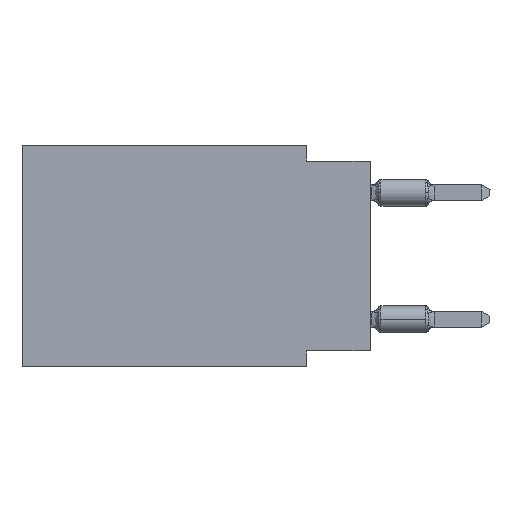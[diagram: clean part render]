
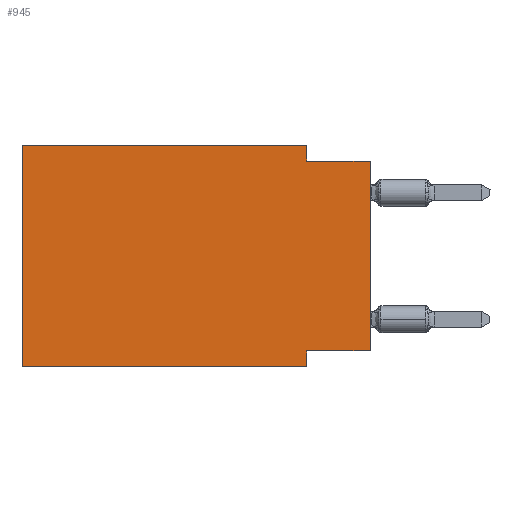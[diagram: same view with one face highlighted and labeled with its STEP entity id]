
A CAD part, left-side view. The second image highlights one B-rep face of the part: STEP entity #945.
In plain terms, the highlighted planar face has unit normal (-1, 0, 0).
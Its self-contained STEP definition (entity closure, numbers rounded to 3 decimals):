
#302 = CARTESIAN_POINT ( 'NONE',  ( 0., 13.97, 0. ) ) ;
#624 = CARTESIAN_POINT ( 'NONE',  ( 0., 0., 0. ) ) ;
#787 = VECTOR ( 'NONE', #10287, 1000. ) ;
#945 = ADVANCED_FACE ( 'NONE', ( #7167 ), #45104, .F. ) ;
#946 = ORIENTED_EDGE ( 'NONE', *, *, #25807, .F. ) ;
#1257 = CARTESIAN_POINT ( 'NONE',  ( 0., 13.97, 0. ) ) ;
#1689 = CARTESIAN_POINT ( 'NONE',  ( 0., 13.97, 0. ) ) ;
#1905 = VERTEX_POINT ( 'NONE', #18632 ) ;
#2307 = ORIENTED_EDGE ( 'NONE', *, *, #4470, .F. ) ;
#2463 = VERTEX_POINT ( 'NONE', #44255 ) ;
#2553 = CARTESIAN_POINT ( 'NONE',  ( 0., 2.54, -8.89 ) ) ;
#2844 = VERTEX_POINT ( 'NONE', #2553 ) ;
#2991 = LINE ( 'NONE', #7091, #787 ) ;
#4079 = EDGE_CURVE ( 'NONE', #14076, #1905, #31933, .T. ) ;
#4213 = ORIENTED_EDGE ( 'NONE', *, *, #28203, .F. ) ;
#4470 = EDGE_CURVE ( 'NONE', #2463, #1905, #44933, .T. ) ;
#4585 = LINE ( 'NONE', #14881, #16093 ) ;
#6773 = DIRECTION ( 'NONE',  ( 0., -1., 0. ) ) ;
#7091 = CARTESIAN_POINT ( 'NONE',  ( 0., 2.54, -8.89 ) ) ;
#7167 = FACE_OUTER_BOUND ( 'NONE', #30741, .T. ) ;
#7671 = DIRECTION ( 'NONE',  ( 0., 0., 1. ) ) ;
#9624 = VECTOR ( 'NONE', #35718, 1000. ) ;
#10287 = DIRECTION ( 'NONE',  ( 0., 0., -1. ) ) ;
#10493 = VECTOR ( 'NONE', #6773, 1000. ) ;
#10556 = VECTOR ( 'NONE', #17988, 1000. ) ;
#11600 = EDGE_CURVE ( 'NONE', #29975, #2844, #30403, .T. ) ;
#11664 = CARTESIAN_POINT ( 'NONE',  ( 0., 0., -8.255 ) ) ;
#14076 = VERTEX_POINT ( 'NONE', #11664 ) ;
#14382 = ORIENTED_EDGE ( 'NONE', *, *, #4079, .T. ) ;
#14881 = CARTESIAN_POINT ( 'NONE',  ( 0., 13.97, 0. ) ) ;
#16093 = VECTOR ( 'NONE', #35660, 1000. ) ;
#16853 = VERTEX_POINT ( 'NONE', #23059 ) ;
#17988 = DIRECTION ( 'NONE',  ( 0., 0., 1. ) ) ;
#18632 = CARTESIAN_POINT ( 'NONE',  ( 0., 0., -0.635 ) ) ;
#18939 = VERTEX_POINT ( 'NONE', #20439 ) ;
#20439 = CARTESIAN_POINT ( 'NONE',  ( 0., 2.54, 0. ) ) ;
#21323 = DIRECTION ( 'NONE',  ( 0., 0., -1. ) ) ;
#21767 = LINE ( 'NONE', #24309, #9624 ) ;
#23059 = CARTESIAN_POINT ( 'NONE',  ( 0., 2.54, -8.255 ) ) ;
#24309 = CARTESIAN_POINT ( 'NONE',  ( 0., 0., -8.255 ) ) ;
#25141 = EDGE_CURVE ( 'NONE', #29975, #31504, #32350, .T. ) ;
#25807 = EDGE_CURVE ( 'NONE', #31504, #18939, #4585, .T. ) ;
#26710 = EDGE_CURVE ( 'NONE', #18939, #2463, #34114, .T. ) ;
#27057 = ORIENTED_EDGE ( 'NONE', *, *, #11600, .T. ) ;
#27412 = CARTESIAN_POINT ( 'NONE',  ( 0., 13.97, -8.89 ) ) ;
#27734 = DIRECTION ( 'NONE',  ( 1., 0., 0. ) ) ;
#27994 = ORIENTED_EDGE ( 'NONE', *, *, #25141, .F. ) ;
#28203 = EDGE_CURVE ( 'NONE', #16853, #2844, #2991, .T. ) ;
#28872 = AXIS2_PLACEMENT_3D ( 'NONE', #302, #27734, #21323 ) ;
#29975 = VERTEX_POINT ( 'NONE', #43553 ) ;
#30403 = LINE ( 'NONE', #27412, #34099 ) ;
#30741 = EDGE_LOOP ( 'NONE', ( #14382, #2307, #41811, #946, #27994, #27057, #4213, #35517 ) ) ;
#31504 = VERTEX_POINT ( 'NONE', #1689 ) ;
#31933 = LINE ( 'NONE', #624, #10556 ) ;
#32350 = LINE ( 'NONE', #1257, #34973 ) ;
#33667 = CARTESIAN_POINT ( 'NONE',  ( 0., 2.54, 0. ) ) ;
#34099 = VECTOR ( 'NONE', #44337, 1000. ) ;
#34114 = LINE ( 'NONE', #33667, #44603 ) ;
#34973 = VECTOR ( 'NONE', #7671, 1000. ) ;
#35081 = CARTESIAN_POINT ( 'NONE',  ( 0., 0., -0.635 ) ) ;
#35517 = ORIENTED_EDGE ( 'NONE', *, *, #35965, .F. ) ;
#35660 = DIRECTION ( 'NONE',  ( 0., -1., 0. ) ) ;
#35718 = DIRECTION ( 'NONE',  ( 0., 1., 0. ) ) ;
#35965 = EDGE_CURVE ( 'NONE', #14076, #16853, #21767, .T. ) ;
#41811 = ORIENTED_EDGE ( 'NONE', *, *, #26710, .F. ) ;
#43553 = CARTESIAN_POINT ( 'NONE',  ( 0., 13.97, -8.89 ) ) ;
#44255 = CARTESIAN_POINT ( 'NONE',  ( 0., 2.54, -0.635 ) ) ;
#44337 = DIRECTION ( 'NONE',  ( 0., -1., 0. ) ) ;
#44397 = DIRECTION ( 'NONE',  ( 0., 0., -1. ) ) ;
#44603 = VECTOR ( 'NONE', #44397, 1000. ) ;
#44933 = LINE ( 'NONE', #35081, #10493 ) ;
#45104 = PLANE ( 'NONE',  #28872 ) ;
